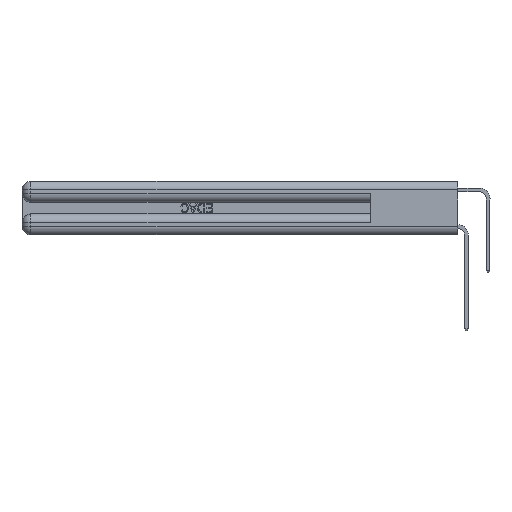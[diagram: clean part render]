
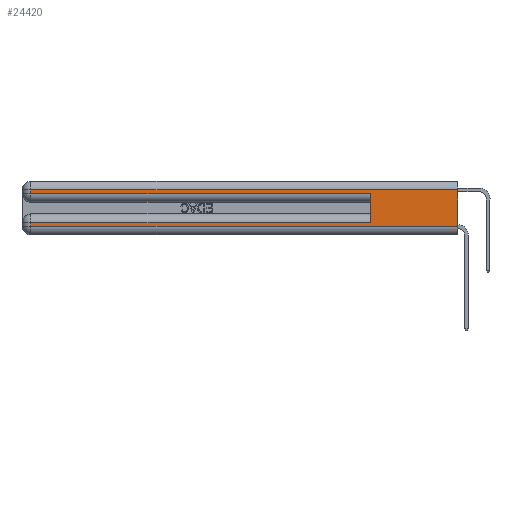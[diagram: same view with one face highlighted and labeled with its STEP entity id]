
A CAD part, left-side view. The second image highlights one B-rep face of the part: STEP entity #24420.
In plain terms, the highlighted planar face has unit normal (-1, 0, 0).
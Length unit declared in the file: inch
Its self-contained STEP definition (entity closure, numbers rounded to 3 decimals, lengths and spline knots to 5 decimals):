
#140 = CARTESIAN_POINT ( 'NONE',  ( 0., 0., 0.085 ) ) ;
#448 = ORIENTED_EDGE ( 'NONE', *, *, #25388, .T. ) ;
#536 = DIRECTION ( 'NONE',  ( 0., 1., 0. ) ) ;
#837 = CARTESIAN_POINT ( 'NONE',  ( 0., 2.94, 0.285 ) ) ;
#895 = PLANE ( 'NONE',  #27104 ) ;
#1139 = CARTESIAN_POINT ( 'NONE',  ( 0., 0., 0.37 ) ) ;
#1539 = VERTEX_POINT ( 'NONE', #837 ) ;
#1634 = VERTEX_POINT ( 'NONE', #18588 ) ;
#1650 = VECTOR ( 'NONE', #19760, 39.37008 ) ;
#1811 = VECTOR ( 'NONE', #2154, 39.37008 ) ;
#2154 = DIRECTION ( 'NONE',  ( 0., -1., 0. ) ) ;
#2703 = VERTEX_POINT ( 'NONE', #19879 ) ;
#4005 = DIRECTION ( 'NONE',  ( 0., 0., -1. ) ) ;
#5283 = LINE ( 'NONE', #28646, #27979 ) ;
#5442 = CARTESIAN_POINT ( 'NONE',  ( 0., 2.94, 0.37 ) ) ;
#7916 = EDGE_CURVE ( 'NONE', #23464, #10669, #19323, .T. ) ;
#8040 = ORIENTED_EDGE ( 'NONE', *, *, #26505, .F. ) ;
#8191 = DIRECTION ( 'NONE',  ( 1., 0., 0. ) ) ;
#8592 = CARTESIAN_POINT ( 'NONE',  ( 0., 2.94, 0.06 ) ) ;
#8968 = VECTOR ( 'NONE', #22953, 39.37008 ) ;
#9110 = DIRECTION ( 'NONE',  ( 0., -1., 0. ) ) ;
#10669 = VERTEX_POINT ( 'NONE', #26913 ) ;
#10724 = EDGE_CURVE ( 'NONE', #2703, #21195, #16422, .T. ) ;
#11193 = EDGE_CURVE ( 'NONE', #28950, #2703, #28160, .T. ) ;
#11269 = CARTESIAN_POINT ( 'NONE',  ( 0., 0.6, 0.285 ) ) ;
#13144 = LINE ( 'NONE', #23956, #1811 ) ;
#13652 = CARTESIAN_POINT ( 'NONE',  ( 0., 0., 0.06 ) ) ;
#14227 = DIRECTION ( 'NONE',  ( 0., 0., 1. ) ) ;
#14526 = EDGE_CURVE ( 'NONE', #28950, #18182, #5283, .T. ) ;
#15318 = CARTESIAN_POINT ( 'NONE',  ( 0., 0., 0.31 ) ) ;
#16275 = ORIENTED_EDGE ( 'NONE', *, *, #11193, .T. ) ;
#16422 = LINE ( 'NONE', #5442, #24756 ) ;
#16843 = ORIENTED_EDGE ( 'NONE', *, *, #10724, .T. ) ;
#17598 = CARTESIAN_POINT ( 'NONE',  ( 0., 0., 0.37 ) ) ;
#18182 = VERTEX_POINT ( 'NONE', #11269 ) ;
#18394 = CARTESIAN_POINT ( 'NONE',  ( 0., 2.94, 0.37 ) ) ;
#18588 = CARTESIAN_POINT ( 'NONE',  ( 0., 0., 0.06 ) ) ;
#19323 = LINE ( 'NONE', #15318, #20064 ) ;
#19760 = DIRECTION ( 'NONE',  ( 0., 1., 0. ) ) ;
#19879 = CARTESIAN_POINT ( 'NONE',  ( 0., 2.94, 0.085 ) ) ;
#20064 = VECTOR ( 'NONE', #536, 39.37008 ) ;
#20257 = CARTESIAN_POINT ( 'NONE',  ( 0., 0.6, 0.085 ) ) ;
#20734 = EDGE_CURVE ( 'NONE', #10669, #1539, #20943, .T. ) ;
#20735 = LINE ( 'NONE', #13652, #30573 ) ;
#20943 = LINE ( 'NONE', #18394, #26229 ) ;
#21195 = VERTEX_POINT ( 'NONE', #8592 ) ;
#22234 = ORIENTED_EDGE ( 'NONE', *, *, #7916, .T. ) ;
#22377 = DIRECTION ( 'NONE',  ( 0., 0., -1. ) ) ;
#22953 = DIRECTION ( 'NONE',  ( 0., 0., -1. ) ) ;
#23063 = CARTESIAN_POINT ( 'NONE',  ( 0., 0., 0.31 ) ) ;
#23464 = VERTEX_POINT ( 'NONE', #23063 ) ;
#23956 = CARTESIAN_POINT ( 'NONE',  ( 0., 0., 0.285 ) ) ;
#24020 = ORIENTED_EDGE ( 'NONE', *, *, #30416, .T. ) ;
#24228 = FACE_OUTER_BOUND ( 'NONE', #25940, .T. ) ;
#24231 = ORIENTED_EDGE ( 'NONE', *, *, #20734, .T. ) ;
#24420 = ADVANCED_FACE ( 'NONE', ( #24228 ), #895, .F. ) ;
#24756 = VECTOR ( 'NONE', #22377, 39.37008 ) ;
#24887 = DIRECTION ( 'NONE',  ( 0., 0., -1. ) ) ;
#25388 = EDGE_CURVE ( 'NONE', #1539, #18182, #13144, .T. ) ;
#25940 = EDGE_LOOP ( 'NONE', ( #8040, #22234, #24231, #448, #26852, #16275, #16843, #24020 ) ) ;
#26229 = VECTOR ( 'NONE', #4005, 39.37008 ) ;
#26505 = EDGE_CURVE ( 'NONE', #23464, #1634, #26758, .T. ) ;
#26758 = LINE ( 'NONE', #1139, #8968 ) ;
#26852 = ORIENTED_EDGE ( 'NONE', *, *, #14526, .F. ) ;
#26913 = CARTESIAN_POINT ( 'NONE',  ( 0., 2.94, 0.31 ) ) ;
#27104 = AXIS2_PLACEMENT_3D ( 'NONE', #17598, #8191, #24887 ) ;
#27979 = VECTOR ( 'NONE', #14227, 39.37008 ) ;
#28160 = LINE ( 'NONE', #140, #1650 ) ;
#28646 = CARTESIAN_POINT ( 'NONE',  ( 0., 0.6, 0.145 ) ) ;
#28950 = VERTEX_POINT ( 'NONE', #20257 ) ;
#30416 = EDGE_CURVE ( 'NONE', #21195, #1634, #20735, .T. ) ;
#30573 = VECTOR ( 'NONE', #9110, 39.37008 ) ;
